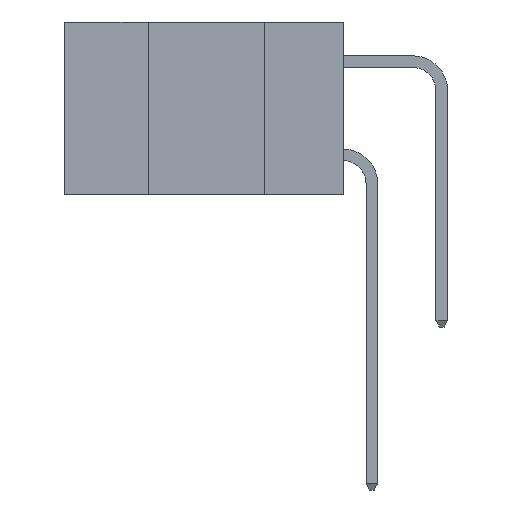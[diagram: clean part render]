
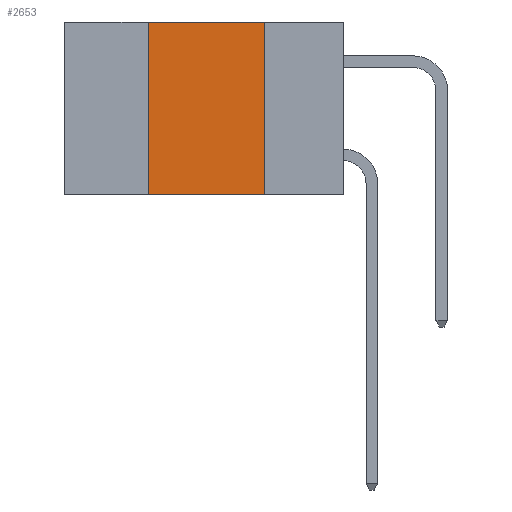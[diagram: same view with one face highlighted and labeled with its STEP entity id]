
A CAD part, left-side view. The second image highlights one B-rep face of the part: STEP entity #2653.
In plain terms, the highlighted planar face has unit normal (-1, 0, 0).
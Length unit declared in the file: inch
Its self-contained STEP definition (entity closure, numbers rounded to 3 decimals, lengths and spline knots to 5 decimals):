
#306 = VERTEX_POINT ( 'NONE', #9905 ) ;
#772 = DIRECTION ( 'NONE',  ( 0., -1., 0. ) ) ;
#1520 = DIRECTION ( 'NONE',  ( 0., 0., 1. ) ) ;
#1616 = ORIENTED_EDGE ( 'NONE', *, *, #10327, .F. ) ;
#2017 = VERTEX_POINT ( 'NONE', #9954 ) ;
#2653 = ADVANCED_FACE ( 'NONE', ( #8197 ), #9102, .F. ) ;
#3463 = VECTOR ( 'NONE', #772, 39.37008 ) ;
#4039 = CARTESIAN_POINT ( 'NONE',  ( 0., 0.17, -0.37 ) ) ;
#4891 = CARTESIAN_POINT ( 'NONE',  ( 0., 0.42, -0.37 ) ) ;
#5603 = DIRECTION ( 'NONE',  ( 0., 0., -1. ) ) ;
#5759 = LINE ( 'NONE', #12377, #11760 ) ;
#6512 = CARTESIAN_POINT ( 'NONE',  ( 0., 0.6, -0.37 ) ) ;
#6620 = ORIENTED_EDGE ( 'NONE', *, *, #11557, .F. ) ;
#7208 = LINE ( 'NONE', #12356, #12850 ) ;
#7234 = VERTEX_POINT ( 'NONE', #4891 ) ;
#7767 = EDGE_LOOP ( 'NONE', ( #6620, #1616, #13673, #8033 ) ) ;
#8033 = ORIENTED_EDGE ( 'NONE', *, *, #10906, .T. ) ;
#8197 = FACE_OUTER_BOUND ( 'NONE', #7767, .T. ) ;
#8348 = CARTESIAN_POINT ( 'NONE',  ( 0., 0.42, -0.37 ) ) ;
#8716 = DIRECTION ( 'NONE',  ( 0., 0., -1. ) ) ;
#8719 = DIRECTION ( 'NONE',  ( 1., 0., 0. ) ) ;
#8815 = CARTESIAN_POINT ( 'NONE',  ( 0., 0.6, 0. ) ) ;
#9102 = PLANE ( 'NONE',  #11098 ) ;
#9470 = VERTEX_POINT ( 'NONE', #4039 ) ;
#9905 = CARTESIAN_POINT ( 'NONE',  ( 0., 0.42, 0. ) ) ;
#9954 = CARTESIAN_POINT ( 'NONE',  ( 0., 0.17, 0. ) ) ;
#10327 = EDGE_CURVE ( 'NONE', #306, #2017, #7208, .T. ) ;
#10610 = EDGE_CURVE ( 'NONE', #7234, #306, #11945, .T. ) ;
#10906 = EDGE_CURVE ( 'NONE', #7234, #9470, #11412, .T. ) ;
#11098 = AXIS2_PLACEMENT_3D ( 'NONE', #8815, #8719, #8716 ) ;
#11412 = LINE ( 'NONE', #6512, #3463 ) ;
#11557 = EDGE_CURVE ( 'NONE', #2017, #9470, #5759, .T. ) ;
#11760 = VECTOR ( 'NONE', #5603, 39.37008 ) ;
#11945 = LINE ( 'NONE', #8348, #12312 ) ;
#12312 = VECTOR ( 'NONE', #1520, 39.37008 ) ;
#12356 = CARTESIAN_POINT ( 'NONE',  ( 0., 0.6, 0. ) ) ;
#12377 = CARTESIAN_POINT ( 'NONE',  ( 0., 0.17, -0.37 ) ) ;
#12850 = VECTOR ( 'NONE', #13482, 39.37008 ) ;
#13482 = DIRECTION ( 'NONE',  ( 0., -1., 0. ) ) ;
#13673 = ORIENTED_EDGE ( 'NONE', *, *, #10610, .F. ) ;
